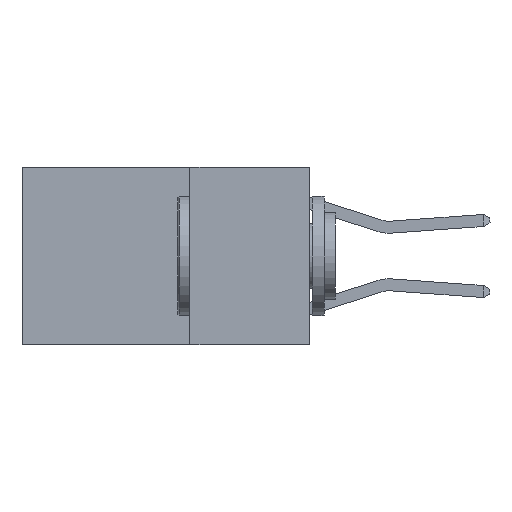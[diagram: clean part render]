
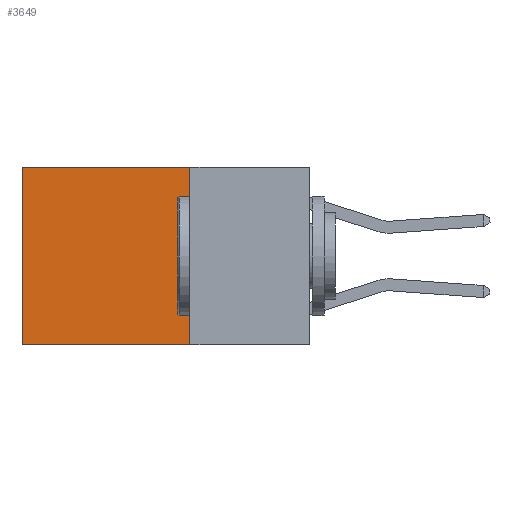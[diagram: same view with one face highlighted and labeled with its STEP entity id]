
A CAD part, left-side view. The second image highlights one B-rep face of the part: STEP entity #3649.
In plain terms, the highlighted planar face has unit normal (-1, 0, 0).
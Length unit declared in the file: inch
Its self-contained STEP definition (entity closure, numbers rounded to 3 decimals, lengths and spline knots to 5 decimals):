
#136 = VERTEX_POINT ( 'NONE', #19725 ) ;
#482 = DIRECTION ( 'NONE',  ( 0., 0., -1. ) ) ;
#1484 = CARTESIAN_POINT ( 'NONE',  ( 0.2625, 0.25, 0. ) ) ;
#2138 = ORIENTED_EDGE ( 'NONE', *, *, #12501, .T. ) ;
#2574 = AXIS2_PLACEMENT_3D ( 'NONE', #12059, #20889, #23522 ) ;
#3649 = ADVANCED_FACE ( 'NONE', ( #22629 ), #9845, .F. ) ;
#6883 = CARTESIAN_POINT ( 'NONE',  ( 0.2625, 0.25, 0. ) ) ;
#7586 = DIRECTION ( 'NONE',  ( 0., 1., 0. ) ) ;
#8467 = VECTOR ( 'NONE', #14014, 39.37008 ) ;
#9792 = LINE ( 'NONE', #14293, #8467 ) ;
#9845 = PLANE ( 'NONE',  #2574 ) ;
#10471 = VERTEX_POINT ( 'NONE', #14964 ) ;
#11739 = EDGE_CURVE ( 'NONE', #16921, #26231, #14751, .T. ) ;
#12014 = CARTESIAN_POINT ( 'NONE',  ( 0.2625, 0.6, 0. ) ) ;
#12059 = CARTESIAN_POINT ( 'NONE',  ( 0.2625, 0.25, 0. ) ) ;
#12501 = EDGE_CURVE ( 'NONE', #26231, #136, #9792, .T. ) ;
#13689 = DIRECTION ( 'NONE',  ( 0., 1., 0. ) ) ;
#14014 = DIRECTION ( 'NONE',  ( 0., 0., -1. ) ) ;
#14293 = CARTESIAN_POINT ( 'NONE',  ( 0.2625, 0.6, 0. ) ) ;
#14751 = LINE ( 'NONE', #1484, #21775 ) ;
#14754 = CARTESIAN_POINT ( 'NONE',  ( 0.2625, 0.25, 0. ) ) ;
#14964 = CARTESIAN_POINT ( 'NONE',  ( 0.2625, 0.25, -0.37 ) ) ;
#15253 = EDGE_CURVE ( 'NONE', #16921, #10471, #23883, .T. ) ;
#16921 = VERTEX_POINT ( 'NONE', #14754 ) ;
#17308 = EDGE_LOOP ( 'NONE', ( #2138, #21331, #19031, #24739 ) ) ;
#17317 = VECTOR ( 'NONE', #13689, 39.37008 ) ;
#17961 = CARTESIAN_POINT ( 'NONE',  ( 0.2625, 0.25, -0.37 ) ) ;
#18176 = VECTOR ( 'NONE', #482, 39.37008 ) ;
#18413 = EDGE_CURVE ( 'NONE', #10471, #136, #23732, .T. ) ;
#19031 = ORIENTED_EDGE ( 'NONE', *, *, #15253, .F. ) ;
#19725 = CARTESIAN_POINT ( 'NONE',  ( 0.2625, 0.6, -0.37 ) ) ;
#20889 = DIRECTION ( 'NONE',  ( 1., 0., 0. ) ) ;
#21331 = ORIENTED_EDGE ( 'NONE', *, *, #18413, .F. ) ;
#21775 = VECTOR ( 'NONE', #7586, 39.37008 ) ;
#22629 = FACE_OUTER_BOUND ( 'NONE', #17308, .T. ) ;
#23522 = DIRECTION ( 'NONE',  ( 0., 0., -1. ) ) ;
#23732 = LINE ( 'NONE', #17961, #17317 ) ;
#23883 = LINE ( 'NONE', #6883, #18176 ) ;
#24739 = ORIENTED_EDGE ( 'NONE', *, *, #11739, .T. ) ;
#26231 = VERTEX_POINT ( 'NONE', #12014 ) ;
